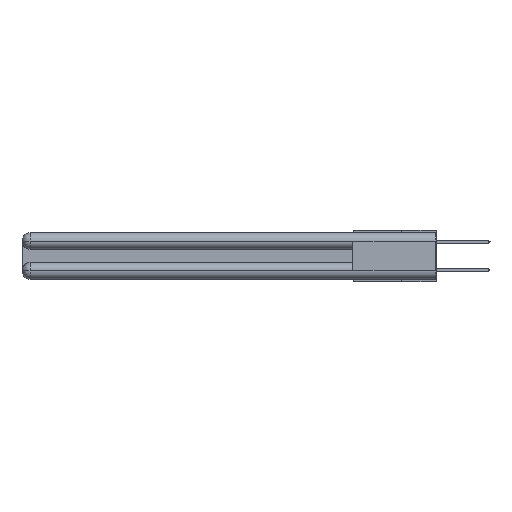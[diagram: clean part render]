
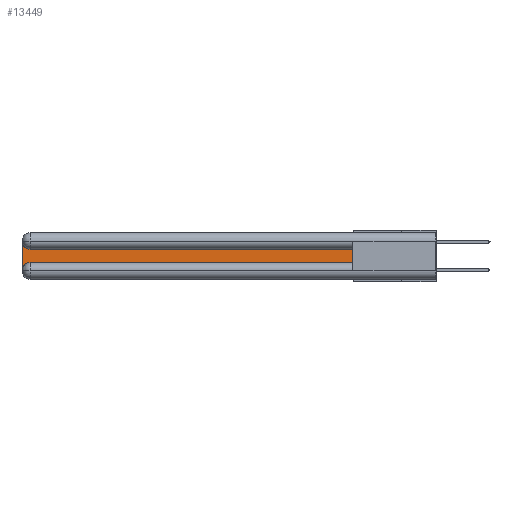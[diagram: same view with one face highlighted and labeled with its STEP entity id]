
A CAD part, left-side view. The second image highlights one B-rep face of the part: STEP entity #13449.
In plain terms, the highlighted planar face has unit normal (-1, 0, 0).
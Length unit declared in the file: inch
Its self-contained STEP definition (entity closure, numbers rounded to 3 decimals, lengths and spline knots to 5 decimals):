
#488 = VERTEX_POINT ( 'NONE', #4786 ) ;
#610 = DIRECTION ( 'NONE',  ( 0., 0., 1. ) ) ;
#1291 = CARTESIAN_POINT ( 'NONE',  ( 0.075, 3., -0.2175 ) ) ;
#1296 = ORIENTED_EDGE ( 'NONE', *, *, #26106, .T. ) ;
#1896 = ORIENTED_EDGE ( 'NONE', *, *, #20392, .T. ) ;
#1910 = EDGE_CURVE ( 'NONE', #10968, #4731, #9334, .T. ) ;
#2275 = CARTESIAN_POINT ( 'NONE',  ( 0.075, 3., -0.2775 ) ) ;
#2407 = LINE ( 'NONE', #6328, #5730 ) ;
#2643 = DIRECTION ( 'NONE',  ( 0., 0., -1. ) ) ;
#3696 = DIRECTION ( 'NONE',  ( 0., 0., -1. ) ) ;
#4246 = PLANE ( 'NONE',  #17133 ) ;
#4485 = VECTOR ( 'NONE', #26687, 39.37008 ) ;
#4519 = AXIS2_PLACEMENT_3D ( 'NONE', #15991, #18114, #9628 ) ;
#4731 = VERTEX_POINT ( 'NONE', #6315 ) ;
#4786 = CARTESIAN_POINT ( 'NONE',  ( 0.075, 2.94, -0.1225 ) ) ;
#5710 = VECTOR ( 'NONE', #610, 39.37008 ) ;
#5730 = VECTOR ( 'NONE', #23212, 39.37008 ) ;
#5779 = VERTEX_POINT ( 'NONE', #2275 ) ;
#6315 = CARTESIAN_POINT ( 'NONE',  ( 0.075, 0.6, -0.1225 ) ) ;
#6328 = CARTESIAN_POINT ( 'NONE',  ( 0.075, 0.6, -0.2175 ) ) ;
#8494 = CARTESIAN_POINT ( 'NONE',  ( 0.075, 3., -0.1225 ) ) ;
#9211 = CARTESIAN_POINT ( 'NONE',  ( 0.075, 0.6, -0.2175 ) ) ;
#9334 = LINE ( 'NONE', #9211, #5710 ) ;
#9628 = DIRECTION ( 'NONE',  ( 0., 0., -1. ) ) ;
#10028 = CARTESIAN_POINT ( 'NONE',  ( 0.075, 2.94, -0.2175 ) ) ;
#10218 = DIRECTION ( 'NONE',  ( 1., 0., 0. ) ) ;
#10772 = CIRCLE ( 'NONE', #11349, 0.06 ) ;
#10968 = VERTEX_POINT ( 'NONE', #23097 ) ;
#11349 = AXIS2_PLACEMENT_3D ( 'NONE', #25058, #10218, #12485 ) ;
#12013 = ORIENTED_EDGE ( 'NONE', *, *, #17413, .T. ) ;
#12485 = DIRECTION ( 'NONE',  ( 0., 0., -1. ) ) ;
#13449 = ADVANCED_FACE ( 'NONE', ( #23466 ), #4246, .F. ) ;
#13609 = EDGE_LOOP ( 'NONE', ( #1296, #1896, #12013, #25680, #26927, #15171 ) ) ;
#14067 = CARTESIAN_POINT ( 'NONE',  ( 0.075, 3., -0.0625 ) ) ;
#14478 = LINE ( 'NONE', #22687, #4485 ) ;
#14526 = VERTEX_POINT ( 'NONE', #14067 ) ;
#14979 = VECTOR ( 'NONE', #3696, 39.37008 ) ;
#15171 = ORIENTED_EDGE ( 'NONE', *, *, #1910, .T. ) ;
#15991 = CARTESIAN_POINT ( 'NONE',  ( 0.075, 2.94, -0.2775 ) ) ;
#17133 = AXIS2_PLACEMENT_3D ( 'NONE', #8494, #23526, #2643 ) ;
#17413 = EDGE_CURVE ( 'NONE', #14526, #5779, #23579, .T. ) ;
#18114 = DIRECTION ( 'NONE',  ( 1., 0., 0. ) ) ;
#19446 = VERTEX_POINT ( 'NONE', #10028 ) ;
#20392 = EDGE_CURVE ( 'NONE', #488, #14526, #10772, .T. ) ;
#22399 = CIRCLE ( 'NONE', #4519, 0.06 ) ;
#22687 = CARTESIAN_POINT ( 'NONE',  ( 0.075, 0.6, -0.1225 ) ) ;
#23097 = CARTESIAN_POINT ( 'NONE',  ( 0.075, 0.6, -0.2175 ) ) ;
#23212 = DIRECTION ( 'NONE',  ( 0., -1., 0. ) ) ;
#23466 = FACE_OUTER_BOUND ( 'NONE', #13609, .T. ) ;
#23526 = DIRECTION ( 'NONE',  ( 1., 0., 0. ) ) ;
#23579 = LINE ( 'NONE', #1291, #14979 ) ;
#25058 = CARTESIAN_POINT ( 'NONE',  ( 0.075, 2.94, -0.0625 ) ) ;
#25680 = ORIENTED_EDGE ( 'NONE', *, *, #25941, .T. ) ;
#25941 = EDGE_CURVE ( 'NONE', #5779, #19446, #22399, .T. ) ;
#26106 = EDGE_CURVE ( 'NONE', #4731, #488, #14478, .T. ) ;
#26687 = DIRECTION ( 'NONE',  ( 0., 1., 0. ) ) ;
#26927 = ORIENTED_EDGE ( 'NONE', *, *, #27288, .T. ) ;
#27288 = EDGE_CURVE ( 'NONE', #19446, #10968, #2407, .T. ) ;
